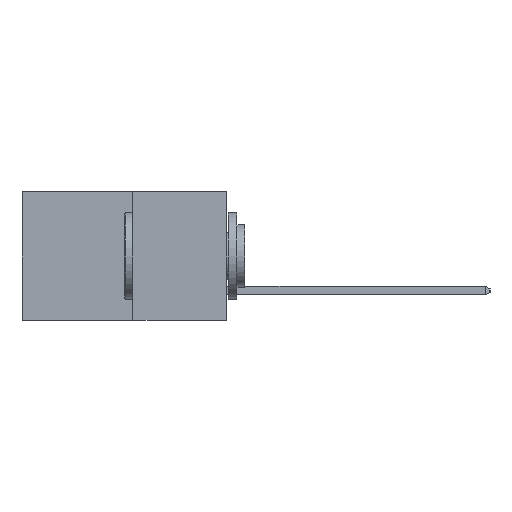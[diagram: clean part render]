
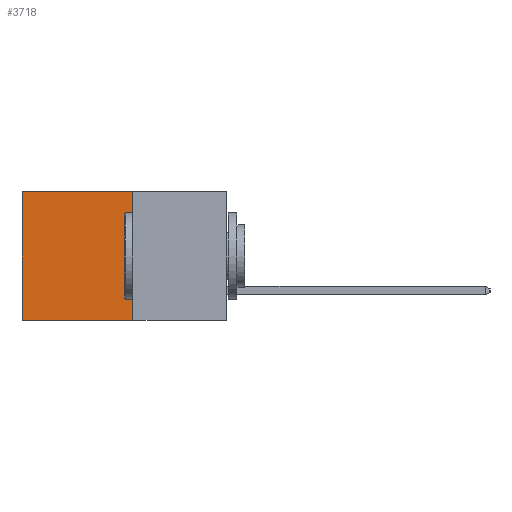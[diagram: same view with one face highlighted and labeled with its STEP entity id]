
A CAD part, left-side view. The second image highlights one B-rep face of the part: STEP entity #3718.
In plain terms, the highlighted planar face has unit normal (-1, 0, 0).
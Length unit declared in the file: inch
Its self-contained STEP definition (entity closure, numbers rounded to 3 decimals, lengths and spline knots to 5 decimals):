
#492 = EDGE_LOOP ( 'NONE', ( #4400, #15413, #4283, #10235 ) ) ;
#1191 = CARTESIAN_POINT ( 'NONE',  ( 0.277, 0.27, -0.37 ) ) ;
#1558 = DIRECTION ( 'NONE',  ( 0., 0., -1. ) ) ;
#3718 = ADVANCED_FACE ( 'NONE', ( #19603 ), #9933, .F. ) ;
#4283 = ORIENTED_EDGE ( 'NONE', *, *, #18849, .F. ) ;
#4400 = ORIENTED_EDGE ( 'NONE', *, *, #18656, .T. ) ;
#7398 = VECTOR ( 'NONE', #21658, 39.37008 ) ;
#7699 = CARTESIAN_POINT ( 'NONE',  ( 0.277, 0.27, -0.37 ) ) ;
#9851 = DIRECTION ( 'NONE',  ( 0., 0., -1. ) ) ;
#9875 = DIRECTION ( 'NONE',  ( 1., 0., 0. ) ) ;
#9933 = PLANE ( 'NONE',  #13968 ) ;
#10176 = VERTEX_POINT ( 'NONE', #24960 ) ;
#10235 = ORIENTED_EDGE ( 'NONE', *, *, #23190, .T. ) ;
#11107 = DIRECTION ( 'NONE',  ( 0., 1., 0. ) ) ;
#13648 = VECTOR ( 'NONE', #1558, 39.37008 ) ;
#13921 = LINE ( 'NONE', #18079, #23695 ) ;
#13968 = AXIS2_PLACEMENT_3D ( 'NONE', #14965, #9875, #9851 ) ;
#14873 = VERTEX_POINT ( 'NONE', #7699 ) ;
#14965 = CARTESIAN_POINT ( 'NONE',  ( 0.277, 0.27, -0.37 ) ) ;
#15413 = ORIENTED_EDGE ( 'NONE', *, *, #22243, .F. ) ;
#15786 = CARTESIAN_POINT ( 'NONE',  ( 0.277, 0.27, 0. ) ) ;
#16446 = VERTEX_POINT ( 'NONE', #24442 ) ;
#17084 = VECTOR ( 'NONE', #11107, 39.37008 ) ;
#18079 = CARTESIAN_POINT ( 'NONE',  ( 0.277, 0.27, -0.37 ) ) ;
#18656 = EDGE_CURVE ( 'NONE', #16446, #22220, #24663, .T. ) ;
#18849 = EDGE_CURVE ( 'NONE', #10176, #14873, #13921, .T. ) ;
#19204 = LINE ( 'NONE', #15786, #7398 ) ;
#19603 = FACE_OUTER_BOUND ( 'NONE', #492, .T. ) ;
#20036 = DIRECTION ( 'NONE',  ( 0., 0., -1. ) ) ;
#21658 = DIRECTION ( 'NONE',  ( 0., 1., 0. ) ) ;
#22220 = VERTEX_POINT ( 'NONE', #24736 ) ;
#22243 = EDGE_CURVE ( 'NONE', #14873, #22220, #22248, .T. ) ;
#22248 = LINE ( 'NONE', #1191, #17084 ) ;
#23190 = EDGE_CURVE ( 'NONE', #10176, #16446, #19204, .T. ) ;
#23695 = VECTOR ( 'NONE', #20036, 39.37008 ) ;
#24442 = CARTESIAN_POINT ( 'NONE',  ( 0.277, 0.59, 0. ) ) ;
#24663 = LINE ( 'NONE', #25171, #13648 ) ;
#24736 = CARTESIAN_POINT ( 'NONE',  ( 0.277, 0.59, -0.37 ) ) ;
#24960 = CARTESIAN_POINT ( 'NONE',  ( 0.277, 0.27, 0. ) ) ;
#25171 = CARTESIAN_POINT ( 'NONE',  ( 0.277, 0.59, -0.37 ) ) ;
